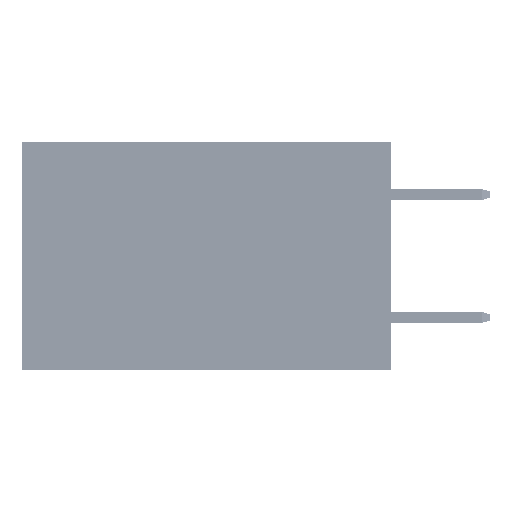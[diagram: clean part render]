
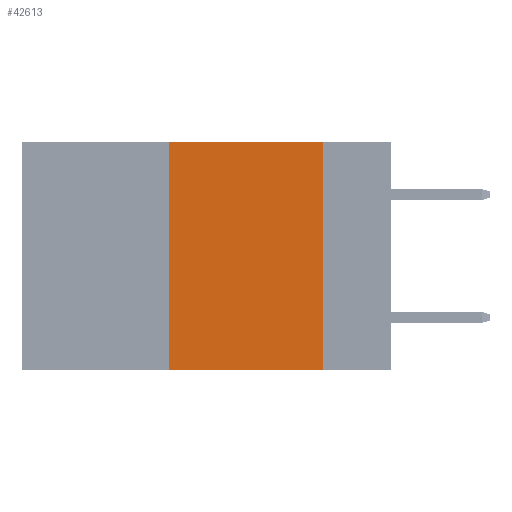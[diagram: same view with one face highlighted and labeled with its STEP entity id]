
A CAD part, left-side view. The second image highlights one B-rep face of the part: STEP entity #42613.
In plain terms, the highlighted planar face has unit normal (-1, 0, 0).
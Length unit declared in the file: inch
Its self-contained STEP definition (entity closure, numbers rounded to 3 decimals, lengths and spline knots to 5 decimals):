
#1280 = LINE ( 'NONE', #26100, #7945 ) ;
#1884 = CARTESIAN_POINT ( 'NONE',  ( 0., 0.6, 0. ) ) ;
#2889 = VERTEX_POINT ( 'NONE', #16898 ) ;
#5648 = VERTEX_POINT ( 'NONE', #10188 ) ;
#7945 = VECTOR ( 'NONE', #33674, 39.37008 ) ;
#10079 = LINE ( 'NONE', #25498, #30896 ) ;
#10187 = EDGE_CURVE ( 'NONE', #2889, #35436, #10079, .T. ) ;
#10188 = CARTESIAN_POINT ( 'NONE',  ( 0., 0.36, 0. ) ) ;
#11731 = VECTOR ( 'NONE', #13370, 39.37008 ) ;
#13370 = DIRECTION ( 'NONE',  ( 0., 0., 1. ) ) ;
#16898 = CARTESIAN_POINT ( 'NONE',  ( 0., 0.36, -0.37 ) ) ;
#19091 = LINE ( 'NONE', #44859, #11731 ) ;
#22336 = AXIS2_PLACEMENT_3D ( 'NONE', #1884, #30220, #41893 ) ;
#23910 = FACE_OUTER_BOUND ( 'NONE', #35530, .T. ) ;
#25498 = CARTESIAN_POINT ( 'NONE',  ( 0., 0.6, -0.37 ) ) ;
#26100 = CARTESIAN_POINT ( 'NONE',  ( 0., 0.6, 0. ) ) ;
#28513 = EDGE_CURVE ( 'NONE', #40711, #35436, #36466, .T. ) ;
#30220 = DIRECTION ( 'NONE',  ( 1., 0., 0. ) ) ;
#30896 = VECTOR ( 'NONE', #40969, 39.37008 ) ;
#32846 = ORIENTED_EDGE ( 'NONE', *, *, #10187, .T. ) ;
#33421 = VECTOR ( 'NONE', #34496, 39.37008 ) ;
#33674 = DIRECTION ( 'NONE',  ( 0., -1., 0. ) ) ;
#34496 = DIRECTION ( 'NONE',  ( 0., 0., -1. ) ) ;
#35436 = VERTEX_POINT ( 'NONE', #38493 ) ;
#35530 = EDGE_LOOP ( 'NONE', ( #45150, #47052, #41706, #32846 ) ) ;
#36466 = LINE ( 'NONE', #50209, #33421 ) ;
#38493 = CARTESIAN_POINT ( 'NONE',  ( 0., 0.11, -0.37 ) ) ;
#40711 = VERTEX_POINT ( 'NONE', #45531 ) ;
#40969 = DIRECTION ( 'NONE',  ( 0., -1., 0. ) ) ;
#41706 = ORIENTED_EDGE ( 'NONE', *, *, #41923, .F. ) ;
#41893 = DIRECTION ( 'NONE',  ( 0., 0., -1. ) ) ;
#41923 = EDGE_CURVE ( 'NONE', #2889, #5648, #19091, .T. ) ;
#42613 = ADVANCED_FACE ( 'NONE', ( #23910 ), #46157, .F. ) ;
#44859 = CARTESIAN_POINT ( 'NONE',  ( 0., 0.36, 0. ) ) ;
#45150 = ORIENTED_EDGE ( 'NONE', *, *, #28513, .F. ) ;
#45218 = EDGE_CURVE ( 'NONE', #5648, #40711, #1280, .T. ) ;
#45531 = CARTESIAN_POINT ( 'NONE',  ( 0., 0.11, 0. ) ) ;
#46157 = PLANE ( 'NONE',  #22336 ) ;
#47052 = ORIENTED_EDGE ( 'NONE', *, *, #45218, .F. ) ;
#50209 = CARTESIAN_POINT ( 'NONE',  ( 0., 0.11, 0. ) ) ;
